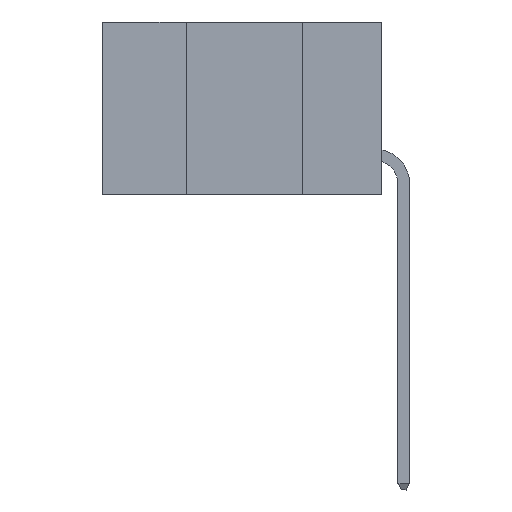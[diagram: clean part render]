
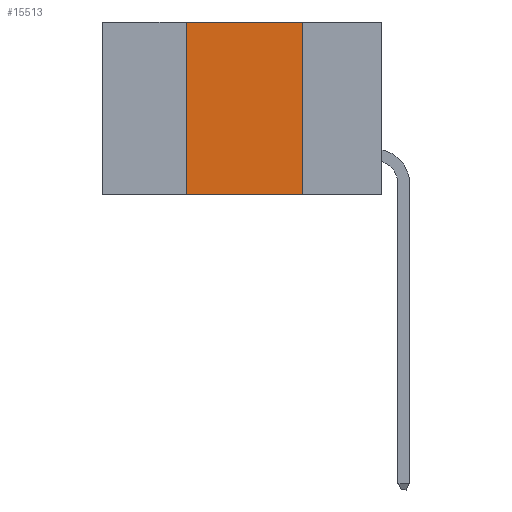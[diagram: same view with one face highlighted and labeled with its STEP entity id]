
A CAD part, left-side view. The second image highlights one B-rep face of the part: STEP entity #15513.
In plain terms, the highlighted planar face has unit normal (-1, 0, 0).
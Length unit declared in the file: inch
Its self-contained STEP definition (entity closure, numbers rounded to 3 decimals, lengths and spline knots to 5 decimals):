
#407 = CARTESIAN_POINT ( 'NONE',  ( 0., 0.17, 0. ) ) ;
#603 = DIRECTION ( 'NONE',  ( 0., 0., -1. ) ) ;
#993 = DIRECTION ( 'NONE',  ( 0., 0., 1. ) ) ;
#1091 = EDGE_LOOP ( 'NONE', ( #2624, #9357, #5963, #3205 ) ) ;
#1119 = CARTESIAN_POINT ( 'NONE',  ( 0., 0.6, -0.37 ) ) ;
#2107 = VECTOR ( 'NONE', #6200, 39.37008 ) ;
#2624 = ORIENTED_EDGE ( 'NONE', *, *, #14522, .F. ) ;
#2700 = VECTOR ( 'NONE', #11020, 39.37008 ) ;
#3205 = ORIENTED_EDGE ( 'NONE', *, *, #17056, .T. ) ;
#3825 = DIRECTION ( 'NONE',  ( 1., 0., 0. ) ) ;
#3862 = VECTOR ( 'NONE', #603, 39.37008 ) ;
#4845 = LINE ( 'NONE', #1119, #2700 ) ;
#5576 = CARTESIAN_POINT ( 'NONE',  ( 0., 0.17, 0. ) ) ;
#5963 = ORIENTED_EDGE ( 'NONE', *, *, #14229, .F. ) ;
#6110 = LINE ( 'NONE', #14604, #2107 ) ;
#6200 = DIRECTION ( 'NONE',  ( 0., -1., 0. ) ) ;
#6758 = CARTESIAN_POINT ( 'NONE',  ( 0., 0.17, -0.37 ) ) ;
#8197 = CARTESIAN_POINT ( 'NONE',  ( 0., 0.42, 0. ) ) ;
#8312 = VERTEX_POINT ( 'NONE', #6758 ) ;
#8451 = CARTESIAN_POINT ( 'NONE',  ( 0., 0.42, 0. ) ) ;
#8714 = AXIS2_PLACEMENT_3D ( 'NONE', #18538, #3825, #15350 ) ;
#9357 = ORIENTED_EDGE ( 'NONE', *, *, #17423, .F. ) ;
#10777 = VECTOR ( 'NONE', #993, 39.37008 ) ;
#11020 = DIRECTION ( 'NONE',  ( 0., -1., 0. ) ) ;
#12537 = VERTEX_POINT ( 'NONE', #8197 ) ;
#12788 = PLANE ( 'NONE',  #8714 ) ;
#12914 = VERTEX_POINT ( 'NONE', #13927 ) ;
#13927 = CARTESIAN_POINT ( 'NONE',  ( 0., 0.42, -0.37 ) ) ;
#14207 = LINE ( 'NONE', #8451, #10777 ) ;
#14229 = EDGE_CURVE ( 'NONE', #12914, #12537, #14207, .T. ) ;
#14522 = EDGE_CURVE ( 'NONE', #18485, #8312, #16362, .T. ) ;
#14604 = CARTESIAN_POINT ( 'NONE',  ( 0., 0.6, 0. ) ) ;
#15350 = DIRECTION ( 'NONE',  ( 0., 0., -1. ) ) ;
#15513 = ADVANCED_FACE ( 'NONE', ( #15523 ), #12788, .F. ) ;
#15523 = FACE_OUTER_BOUND ( 'NONE', #1091, .T. ) ;
#16362 = LINE ( 'NONE', #407, #3862 ) ;
#17056 = EDGE_CURVE ( 'NONE', #12914, #8312, #4845, .T. ) ;
#17423 = EDGE_CURVE ( 'NONE', #12537, #18485, #6110, .T. ) ;
#18485 = VERTEX_POINT ( 'NONE', #5576 ) ;
#18538 = CARTESIAN_POINT ( 'NONE',  ( 0., 0.6, 0. ) ) ;
